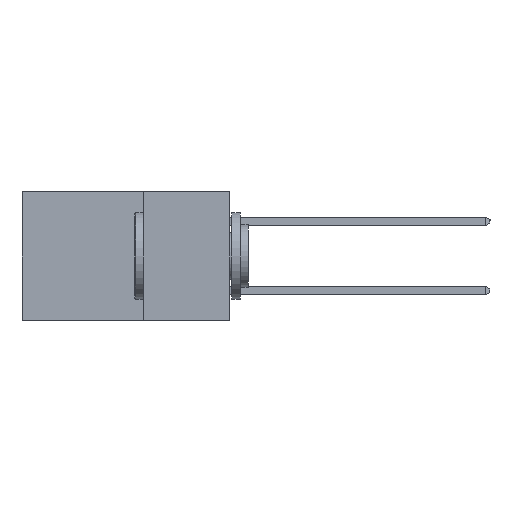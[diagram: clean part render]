
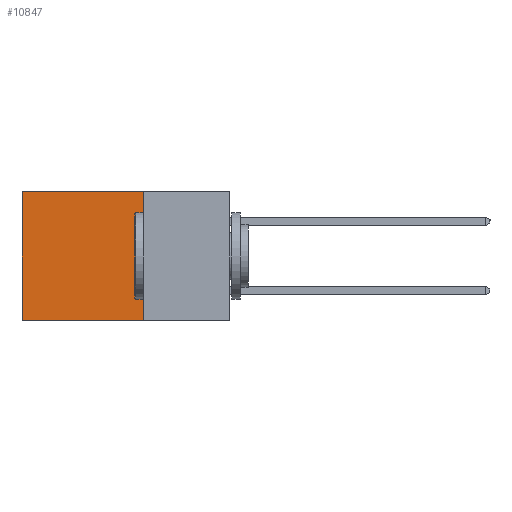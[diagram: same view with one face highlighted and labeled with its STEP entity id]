
A CAD part, left-side view. The second image highlights one B-rep face of the part: STEP entity #10847.
In plain terms, the highlighted planar face has unit normal (-1, 0, 0).
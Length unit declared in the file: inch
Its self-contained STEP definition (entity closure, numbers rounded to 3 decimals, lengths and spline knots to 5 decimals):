
#46 = VECTOR ( 'NONE', #8753, 39.37008 ) ;
#373 = LINE ( 'NONE', #13762, #5350 ) ;
#1789 = DIRECTION ( 'NONE',  ( 0., 1., 0. ) ) ;
#2100 = CARTESIAN_POINT ( 'NONE',  ( 0.2615, 0.6, -0.37 ) ) ;
#2182 = DIRECTION ( 'NONE',  ( 0., 0., -1. ) ) ;
#3132 = CARTESIAN_POINT ( 'NONE',  ( 0.2615, 0.25, 0. ) ) ;
#3872 = DIRECTION ( 'NONE',  ( 0., 0., -1. ) ) ;
#4158 = CARTESIAN_POINT ( 'NONE',  ( 0.2615, 0.25, -0.37 ) ) ;
#5350 = VECTOR ( 'NONE', #3872, 39.37008 ) ;
#5471 = EDGE_CURVE ( 'NONE', #16074, #8510, #14174, .T. ) ;
#6032 = VECTOR ( 'NONE', #12454, 39.37008 ) ;
#7383 = EDGE_CURVE ( 'NONE', #16074, #12651, #14687, .T. ) ;
#8510 = VERTEX_POINT ( 'NONE', #15381 ) ;
#8516 = VECTOR ( 'NONE', #1789, 39.37008 ) ;
#8753 = DIRECTION ( 'NONE',  ( 0., 0., -1. ) ) ;
#8966 = EDGE_CURVE ( 'NONE', #8510, #20953, #15245, .T. ) ;
#10847 = ADVANCED_FACE ( 'NONE', ( #13819 ), #18827, .F. ) ;
#11786 = EDGE_CURVE ( 'NONE', #12651, #20953, #373, .T. ) ;
#11854 = CARTESIAN_POINT ( 'NONE',  ( 0.2615, 0.6, 0. ) ) ;
#12294 = DIRECTION ( 'NONE',  ( 1., 0., 0. ) ) ;
#12454 = DIRECTION ( 'NONE',  ( 0., 1., 0. ) ) ;
#12651 = VERTEX_POINT ( 'NONE', #11854 ) ;
#13418 = CARTESIAN_POINT ( 'NONE',  ( 0.2615, 0.25, -0.37 ) ) ;
#13427 = ORIENTED_EDGE ( 'NONE', *, *, #8966, .F. ) ;
#13762 = CARTESIAN_POINT ( 'NONE',  ( 0.2615, 0.6, -0.37 ) ) ;
#13819 = FACE_OUTER_BOUND ( 'NONE', #18572, .T. ) ;
#14174 = LINE ( 'NONE', #17018, #46 ) ;
#14687 = LINE ( 'NONE', #21384, #6032 ) ;
#15245 = LINE ( 'NONE', #13418, #8516 ) ;
#15381 = CARTESIAN_POINT ( 'NONE',  ( 0.2615, 0.25, -0.37 ) ) ;
#15804 = ORIENTED_EDGE ( 'NONE', *, *, #11786, .T. ) ;
#16074 = VERTEX_POINT ( 'NONE', #3132 ) ;
#16777 = AXIS2_PLACEMENT_3D ( 'NONE', #4158, #12294, #2182 ) ;
#17018 = CARTESIAN_POINT ( 'NONE',  ( 0.2615, 0.25, -0.37 ) ) ;
#17217 = ORIENTED_EDGE ( 'NONE', *, *, #7383, .T. ) ;
#18572 = EDGE_LOOP ( 'NONE', ( #15804, #13427, #19148, #17217 ) ) ;
#18827 = PLANE ( 'NONE',  #16777 ) ;
#19148 = ORIENTED_EDGE ( 'NONE', *, *, #5471, .F. ) ;
#20953 = VERTEX_POINT ( 'NONE', #2100 ) ;
#21384 = CARTESIAN_POINT ( 'NONE',  ( 0.2615, 0.25, 0. ) ) ;
